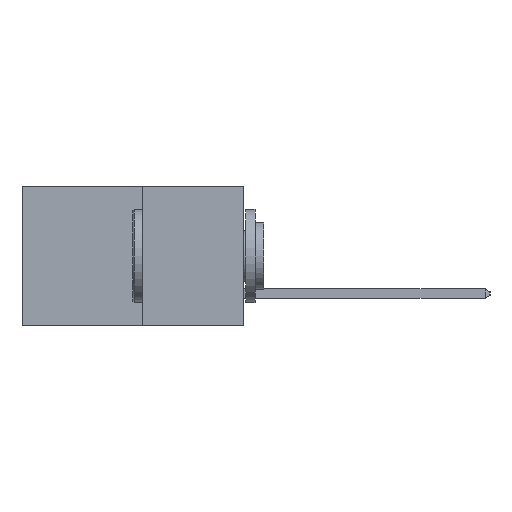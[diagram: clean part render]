
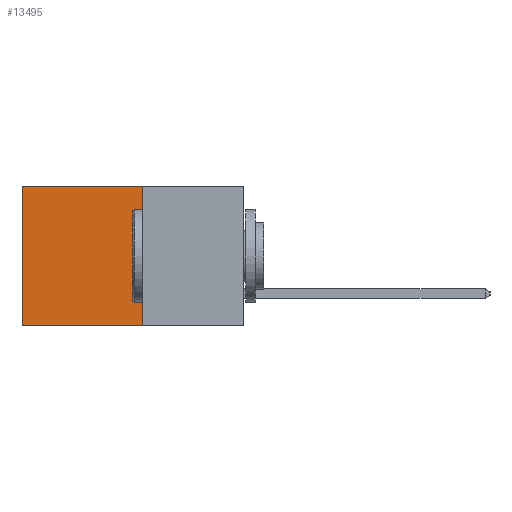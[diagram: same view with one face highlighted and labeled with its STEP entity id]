
A CAD part, left-side view. The second image highlights one B-rep face of the part: STEP entity #13495.
In plain terms, the highlighted planar face has unit normal (-1, 0, 0).
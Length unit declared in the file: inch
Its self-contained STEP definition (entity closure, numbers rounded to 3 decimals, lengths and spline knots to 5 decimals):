
#232 = EDGE_CURVE ( 'NONE', #15257, #11810, #22401, .T. ) ;
#450 = PLANE ( 'NONE',  #2422 ) ;
#1015 = CARTESIAN_POINT ( 'NONE',  ( 0.277, 0.59, -0.37 ) ) ;
#1072 = LINE ( 'NONE', #17336, #5547 ) ;
#1735 = EDGE_CURVE ( 'NONE', #10364, #3894, #8934, .T. ) ;
#2373 = DIRECTION ( 'NONE',  ( 0., 0., -1. ) ) ;
#2422 = AXIS2_PLACEMENT_3D ( 'NONE', #9965, #13745, #2373 ) ;
#2542 = FACE_OUTER_BOUND ( 'NONE', #15172, .T. ) ;
#2868 = VECTOR ( 'NONE', #19118, 39.37008 ) ;
#3894 = VERTEX_POINT ( 'NONE', #22550 ) ;
#4074 = CARTESIAN_POINT ( 'NONE',  ( 0.277, 0.27, 0. ) ) ;
#4162 = CARTESIAN_POINT ( 'NONE',  ( 0.277, 0.27, 0. ) ) ;
#5382 = CARTESIAN_POINT ( 'NONE',  ( 0.277, 0.59, 0. ) ) ;
#5547 = VECTOR ( 'NONE', #13668, 39.37008 ) ;
#7924 = LINE ( 'NONE', #4074, #2868 ) ;
#8500 = EDGE_CURVE ( 'NONE', #10364, #15257, #7924, .T. ) ;
#8934 = LINE ( 'NONE', #22746, #23173 ) ;
#9784 = ORIENTED_EDGE ( 'NONE', *, *, #8500, .T. ) ;
#9965 = CARTESIAN_POINT ( 'NONE',  ( 0.277, 0.27, -0.37 ) ) ;
#10364 = VERTEX_POINT ( 'NONE', #4162 ) ;
#10629 = ORIENTED_EDGE ( 'NONE', *, *, #1735, .F. ) ;
#11810 = VERTEX_POINT ( 'NONE', #1015 ) ;
#12559 = VECTOR ( 'NONE', #23295, 39.37008 ) ;
#12967 = EDGE_CURVE ( 'NONE', #3894, #11810, #1072, .T. ) ;
#13495 = ADVANCED_FACE ( 'NONE', ( #2542 ), #450, .F. ) ;
#13543 = ORIENTED_EDGE ( 'NONE', *, *, #232, .T. ) ;
#13668 = DIRECTION ( 'NONE',  ( 0., 1., 0. ) ) ;
#13745 = DIRECTION ( 'NONE',  ( 1., 0., 0. ) ) ;
#14831 = ORIENTED_EDGE ( 'NONE', *, *, #12967, .F. ) ;
#15172 = EDGE_LOOP ( 'NONE', ( #13543, #14831, #10629, #9784 ) ) ;
#15257 = VERTEX_POINT ( 'NONE', #5382 ) ;
#17336 = CARTESIAN_POINT ( 'NONE',  ( 0.277, 0.27, -0.37 ) ) ;
#18946 = CARTESIAN_POINT ( 'NONE',  ( 0.277, 0.59, -0.37 ) ) ;
#19118 = DIRECTION ( 'NONE',  ( 0., 1., 0. ) ) ;
#19670 = DIRECTION ( 'NONE',  ( 0., 0., -1. ) ) ;
#22401 = LINE ( 'NONE', #18946, #12559 ) ;
#22550 = CARTESIAN_POINT ( 'NONE',  ( 0.277, 0.27, -0.37 ) ) ;
#22746 = CARTESIAN_POINT ( 'NONE',  ( 0.277, 0.27, -0.37 ) ) ;
#23173 = VECTOR ( 'NONE', #19670, 39.37008 ) ;
#23295 = DIRECTION ( 'NONE',  ( 0., 0., -1. ) ) ;
